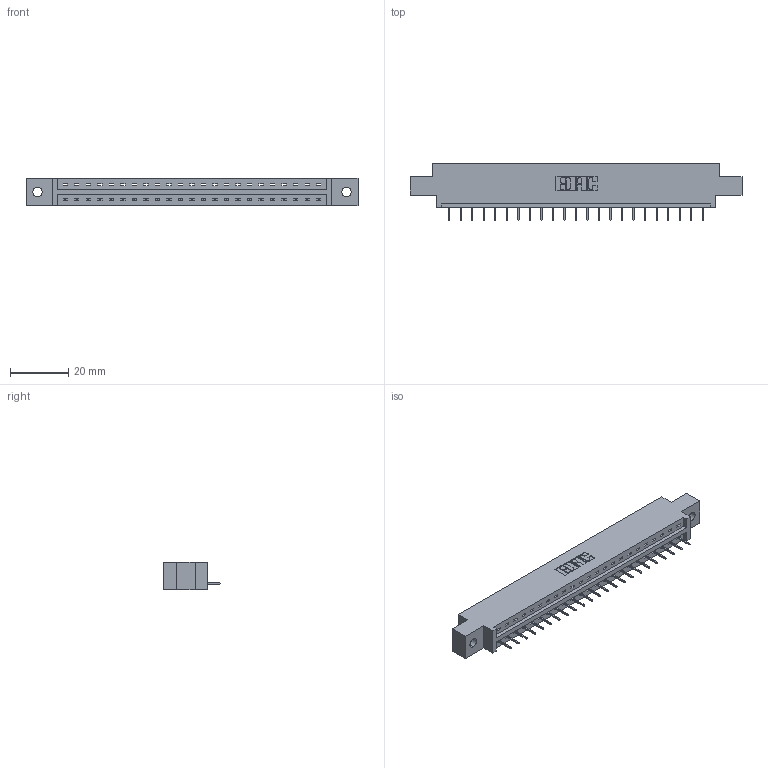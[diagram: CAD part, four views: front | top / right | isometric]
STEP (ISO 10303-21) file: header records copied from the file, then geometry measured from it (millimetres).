
FILE_DESCRIPTION (( 'STEP AP203' ), '1' );
FILE_NAME ('337-023-524-602.STEP', '2018-08-05T16:49:23', ( '' ), ( '' ), 'SwSTEP 2.0', 'SolidWorks 2016', '' );
FILE_SCHEMA (( 'CONFIG_CONTROL_DESIGN' ));
Length unit declared in the file: inch
Products named in the file (3): 337-023-524-602; 337 Part_0.170 Offset - 0.128 Dia; 345-292-001_345-293-124
Assembly tree (24 placements, depth 2):
  337-023-524-602
    337 Part_0.170 Offset - 0.128 Dia
    345-292-001_345-293-124  x23
Bounding box: 114.15 x 19.69 x 9.4 mm (x, y, z)
Volume: 11380.9 mm3; surface area: 11162.1 mm2
Topology: 24 solids, 24 shells, 1636 faces, 4739 edges, 3066 vertices
Faces by surface type: plane 1270, cylinder 366
Entity records: 19763 total; most frequent: CARTESIAN_POINT 3447, ORIENTED_EDGE 3406, DIRECTION 2941, EDGE_CURVE 1703, LINE 1579, VECTOR 1579, VERTEX_POINT 1130, AXIS2_PLACEMENT_3D 681
